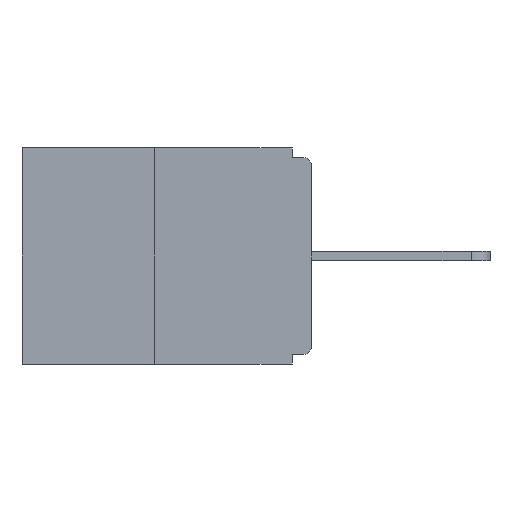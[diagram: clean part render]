
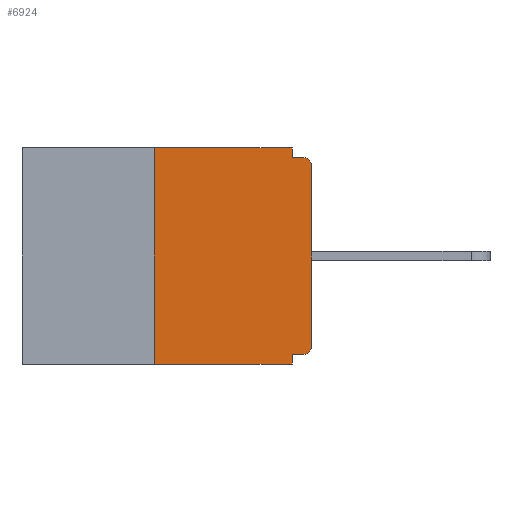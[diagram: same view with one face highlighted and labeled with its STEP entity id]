
A CAD part, left-side view. The second image highlights one B-rep face of the part: STEP entity #6924.
In plain terms, the highlighted planar face has unit normal (-1, 0, 0).
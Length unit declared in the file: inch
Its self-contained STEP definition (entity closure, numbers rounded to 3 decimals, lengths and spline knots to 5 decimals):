
#506 = EDGE_CURVE ( 'NONE', #11166, #3862, #13561, .T. ) ;
#604 = ORIENTED_EDGE ( 'NONE', *, *, #8153, .F. ) ;
#1064 = CARTESIAN_POINT ( 'NONE',  ( 0., 0.031, -0.343 ) ) ;
#1295 = DIRECTION ( 'NONE',  ( 0., 0., -1. ) ) ;
#1309 = DIRECTION ( 'NONE',  ( -1., 0., 0. ) ) ;
#1316 = CARTESIAN_POINT ( 'NONE',  ( 0., 0.25, 0. ) ) ;
#1328 = ORIENTED_EDGE ( 'NONE', *, *, #506, .T. ) ;
#1408 = CARTESIAN_POINT ( 'NONE',  ( 0., 0.015, -0.313 ) ) ;
#1675 = CARTESIAN_POINT ( 'NONE',  ( 0., 0.031, 0. ) ) ;
#2261 = CARTESIAN_POINT ( 'NONE',  ( 0., 0.015, -0.015 ) ) ;
#2756 = LINE ( 'NONE', #7545, #11558 ) ;
#2812 = VECTOR ( 'NONE', #11034, 39.37008 ) ;
#2839 = ORIENTED_EDGE ( 'NONE', *, *, #8543, .T. ) ;
#2928 = DIRECTION ( 'NONE',  ( 0., -1., 0. ) ) ;
#2979 = CARTESIAN_POINT ( 'NONE',  ( 0., 0., -0.328 ) ) ;
#3427 = VERTEX_POINT ( 'NONE', #2261 ) ;
#3439 = CARTESIAN_POINT ( 'NONE',  ( 0., 0., -0.015 ) ) ;
#3469 = DIRECTION ( 'NONE',  ( -1., 0., 0. ) ) ;
#3701 = VERTEX_POINT ( 'NONE', #12168 ) ;
#3774 = VERTEX_POINT ( 'NONE', #9716 ) ;
#3862 = VERTEX_POINT ( 'NONE', #4064 ) ;
#4064 = CARTESIAN_POINT ( 'NONE',  ( 0., 0., -0.313 ) ) ;
#4101 = VERTEX_POINT ( 'NONE', #8623 ) ;
#4494 = ORIENTED_EDGE ( 'NONE', *, *, #12707, .F. ) ;
#4849 = LINE ( 'NONE', #6641, #7598 ) ;
#4888 = CARTESIAN_POINT ( 'NONE',  ( 0., 0., 0. ) ) ;
#5244 = DIRECTION ( 'NONE',  ( 0., -1., 0. ) ) ;
#5827 = ORIENTED_EDGE ( 'NONE', *, *, #10454, .F. ) ;
#6047 = DIRECTION ( 'NONE',  ( 0., 0., -1. ) ) ;
#6137 = DIRECTION ( 'NONE',  ( 1., 0., 0. ) ) ;
#6187 = CARTESIAN_POINT ( 'NONE',  ( 0., 0.46, 0. ) ) ;
#6641 = CARTESIAN_POINT ( 'NONE',  ( 0., 0.46, -0.343 ) ) ;
#6924 = ADVANCED_FACE ( 'NONE', ( #7642 ), #7946, .F. ) ;
#7029 = VERTEX_POINT ( 'NONE', #7050 ) ;
#7050 = CARTESIAN_POINT ( 'NONE',  ( 0., 0.031, -0.015 ) ) ;
#7274 = AXIS2_PLACEMENT_3D ( 'NONE', #6187, #6137, #6047 ) ;
#7545 = CARTESIAN_POINT ( 'NONE',  ( 0., 0.46, 0. ) ) ;
#7598 = VECTOR ( 'NONE', #7864, 39.37008 ) ;
#7609 = AXIS2_PLACEMENT_3D ( 'NONE', #10400, #3469, #11481 ) ;
#7642 = FACE_OUTER_BOUND ( 'NONE', #12212, .T. ) ;
#7864 = DIRECTION ( 'NONE',  ( 0., -1., 0. ) ) ;
#7946 = PLANE ( 'NONE',  #7274 ) ;
#7957 = EDGE_CURVE ( 'NONE', #7029, #3427, #11795, .T. ) ;
#8153 = EDGE_CURVE ( 'NONE', #11166, #14494, #14545, .T. ) ;
#8242 = EDGE_CURVE ( 'NONE', #3774, #11677, #4849, .T. ) ;
#8294 = VERTEX_POINT ( 'NONE', #10188 ) ;
#8543 = EDGE_CURVE ( 'NONE', #3862, #3701, #12296, .T. ) ;
#8623 = CARTESIAN_POINT ( 'NONE',  ( 0., 0.25, 0. ) ) ;
#8781 = VECTOR ( 'NONE', #10074, 39.37008 ) ;
#8875 = VECTOR ( 'NONE', #2928, 39.37008 ) ;
#8955 = CARTESIAN_POINT ( 'NONE',  ( 0., 0.031, -0.343 ) ) ;
#9716 = CARTESIAN_POINT ( 'NONE',  ( 0., 0.25, -0.343 ) ) ;
#10030 = CIRCLE ( 'NONE', #7609, 0.015 ) ;
#10074 = DIRECTION ( 'NONE',  ( 0., 0., -1. ) ) ;
#10188 = CARTESIAN_POINT ( 'NONE',  ( 0., 0.031, 0. ) ) ;
#10400 = CARTESIAN_POINT ( 'NONE',  ( 0., 0.015, -0.03 ) ) ;
#10454 = EDGE_CURVE ( 'NONE', #8294, #7029, #14817, .T. ) ;
#10460 = EDGE_CURVE ( 'NONE', #4101, #8294, #2756, .T. ) ;
#10752 = EDGE_CURVE ( 'NONE', #3701, #3427, #10030, .T. ) ;
#10919 = DIRECTION ( 'NONE',  ( 0., 0., -1. ) ) ;
#11034 = DIRECTION ( 'NONE',  ( 0., 1., 0. ) ) ;
#11166 = VERTEX_POINT ( 'NONE', #11531 ) ;
#11395 = ORIENTED_EDGE ( 'NONE', *, *, #10460, .F. ) ;
#11466 = AXIS2_PLACEMENT_3D ( 'NONE', #1408, #1309, #1295 ) ;
#11481 = DIRECTION ( 'NONE',  ( 0., 0., -1. ) ) ;
#11531 = CARTESIAN_POINT ( 'NONE',  ( 0., 0.015, -0.328 ) ) ;
#11558 = VECTOR ( 'NONE', #5244, 39.37008 ) ;
#11595 = VECTOR ( 'NONE', #13930, 39.37008 ) ;
#11677 = VERTEX_POINT ( 'NONE', #1064 ) ;
#11778 = ORIENTED_EDGE ( 'NONE', *, *, #12433, .F. ) ;
#11795 = LINE ( 'NONE', #3439, #8875 ) ;
#12168 = CARTESIAN_POINT ( 'NONE',  ( 0., 0., -0.03 ) ) ;
#12212 = EDGE_LOOP ( 'NONE', ( #11395, #11778, #13893, #4494, #604, #1328, #2839, #14046, #12840, #5827 ) ) ;
#12296 = LINE ( 'NONE', #4888, #11595 ) ;
#12433 = EDGE_CURVE ( 'NONE', #3774, #4101, #13264, .T. ) ;
#12552 = CARTESIAN_POINT ( 'NONE',  ( 0., 0.031, -0.328 ) ) ;
#12707 = EDGE_CURVE ( 'NONE', #14494, #11677, #14630, .T. ) ;
#12840 = ORIENTED_EDGE ( 'NONE', *, *, #7957, .F. ) ;
#12928 = VECTOR ( 'NONE', #13875, 39.37008 ) ;
#13264 = LINE ( 'NONE', #1316, #12928 ) ;
#13561 = CIRCLE ( 'NONE', #11466, 0.015 ) ;
#13875 = DIRECTION ( 'NONE',  ( 0., 0., 1. ) ) ;
#13893 = ORIENTED_EDGE ( 'NONE', *, *, #8242, .T. ) ;
#13930 = DIRECTION ( 'NONE',  ( 0., 0., 1. ) ) ;
#14046 = ORIENTED_EDGE ( 'NONE', *, *, #10752, .T. ) ;
#14170 = VECTOR ( 'NONE', #10919, 39.37008 ) ;
#14494 = VERTEX_POINT ( 'NONE', #12552 ) ;
#14545 = LINE ( 'NONE', #2979, #2812 ) ;
#14630 = LINE ( 'NONE', #8955, #8781 ) ;
#14817 = LINE ( 'NONE', #1675, #14170 ) ;
